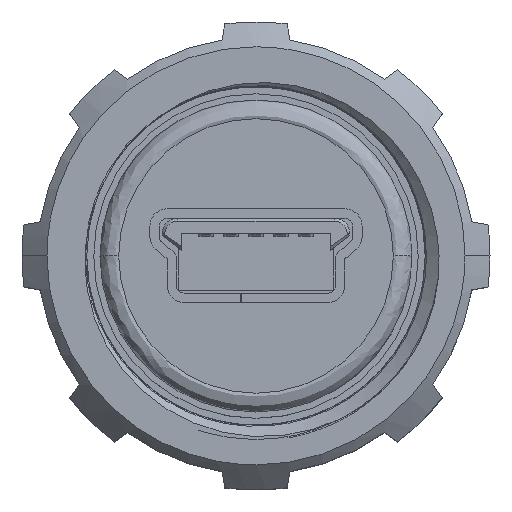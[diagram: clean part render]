
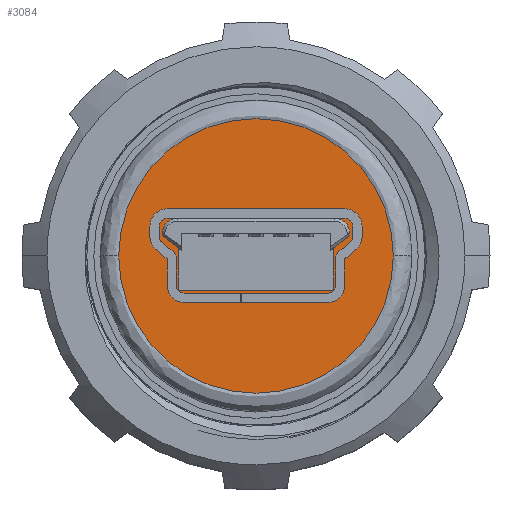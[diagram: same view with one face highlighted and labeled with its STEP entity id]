
A CAD part, top view. The second image highlights one B-rep face of the part: STEP entity #3084.
In plain terms, the highlighted face is planar.
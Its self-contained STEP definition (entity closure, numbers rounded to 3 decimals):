
#405 = CARTESIAN_POINT ( 'NONE',  ( 0., 0., 0. ) ) ;
#2053 = ORIENTED_EDGE ( 'NONE', *, *, #19550, .F. ) ;
#2372 = PLANE ( 'NONE',  #10642 ) ;
#2386 = DIRECTION ( 'NONE',  ( 1., 0., 0. ) ) ;
#3084 = ADVANCED_FACE ( 'NONE', ( #11748 ), #2372, .F. ) ;
#6070 = CARTESIAN_POINT ( 'NONE',  ( 0., 0., 0. ) ) ;
#6128 = DIRECTION ( 'NONE',  ( 0., 0., -1. ) ) ;
#7279 = CARTESIAN_POINT ( 'NONE',  ( 0., 0., -4.4 ) ) ;
#7657 = ORIENTED_EDGE ( 'NONE', *, *, #12145, .F. ) ;
#7709 = DIRECTION ( 'NONE',  ( 1., 0., 0. ) ) ;
#9520 = DIRECTION ( 'NONE',  ( 1., 0., 0. ) ) ;
#10495 = VERTEX_POINT ( 'NONE', #7279 ) ;
#10642 = AXIS2_PLACEMENT_3D ( 'NONE', #16869, #9520, #6128 ) ;
#11748 = FACE_OUTER_BOUND ( 'NONE', #14164, .T. ) ;
#12145 = EDGE_CURVE ( 'NONE', #10495, #15130, #22400, .T. ) ;
#14164 = EDGE_LOOP ( 'NONE', ( #7657, #2053 ) ) ;
#14982 = AXIS2_PLACEMENT_3D ( 'NONE', #405, #2386, #20192 ) ;
#15130 = VERTEX_POINT ( 'NONE', #19232 ) ;
#16869 = CARTESIAN_POINT ( 'NONE',  ( 0., 0., 0. ) ) ;
#18654 = AXIS2_PLACEMENT_3D ( 'NONE', #6070, #7709, #20703 ) ;
#19232 = CARTESIAN_POINT ( 'NONE',  ( 0., 0., 4.4 ) ) ;
#19550 = EDGE_CURVE ( 'NONE', #15130, #10495, #19900, .T. ) ;
#19900 = CIRCLE ( 'NONE', #14982, 4.4 ) ;
#20192 = DIRECTION ( 'NONE',  ( 0., 0., -1. ) ) ;
#20703 = DIRECTION ( 'NONE',  ( 0., 0., -1. ) ) ;
#22400 = CIRCLE ( 'NONE', #18654, 4.4 ) ;
